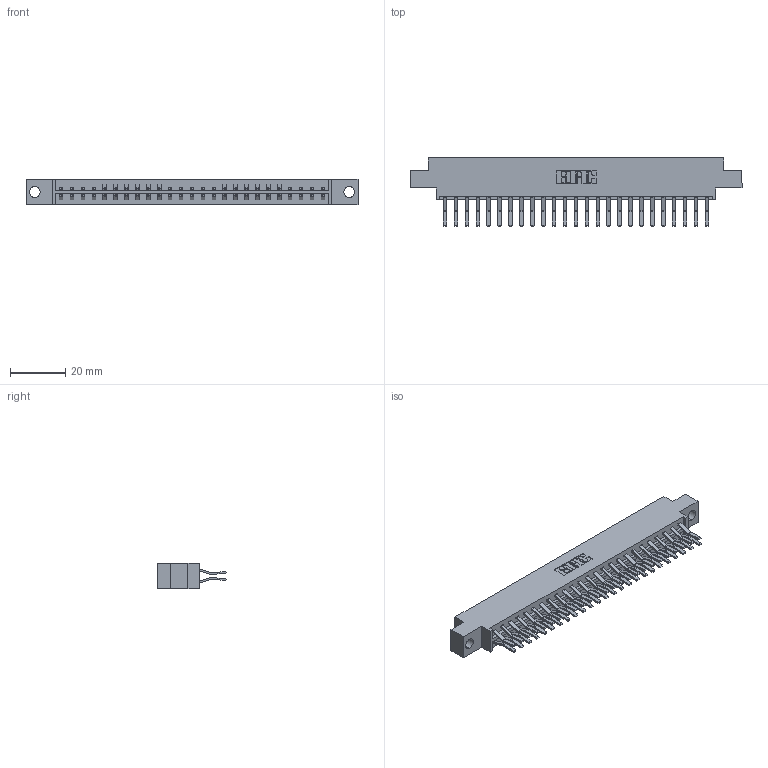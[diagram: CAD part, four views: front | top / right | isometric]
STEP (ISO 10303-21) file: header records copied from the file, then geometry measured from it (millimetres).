
FILE_DESCRIPTION (( 'STEP AP203' ), '1' );
FILE_NAME ('333-050-560-804.STEP', '2018-08-04T01:40:35', ( '' ), ( '' ), 'SwSTEP 2.0', 'SolidWorks 2016', '' );
FILE_SCHEMA (( 'CONFIG_CONTROL_DESIGN' ));
Length unit declared in the file: inch
Products named in the file (3): 345-292-001_560 Tail; 333-050-560-804; 333 Part_Offset - .156 Dia - TH
Assembly tree (51 placements, depth 2):
  333-050-560-804
    333 Part_Offset - .156 Dia - TH
    345-292-001_560 Tail  x50
Bounding box: 120.6 x 24.78 x 9.4 mm (x, y, z)
Volume: 12165.6 mm3; surface area: 15155.2 mm2
Topology: 51 solids, 51 shells, 2818 faces, 8373 edges, 5514 vertices
Faces by surface type: plane 1874, cylinder 944
Entity records: 18505 total; most frequent: CARTESIAN_POINT 3090, ORIENTED_EDGE 3026, DIRECTION 2673, EDGE_CURVE 1513, LINE 1381, VECTOR 1381, VERTEX_POINT 1006, AXIS2_PLACEMENT_3D 646
